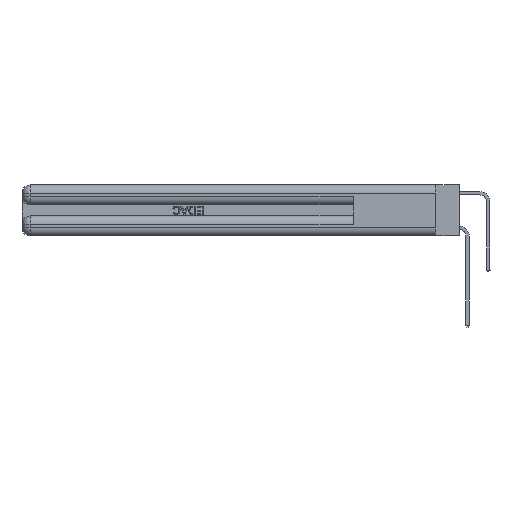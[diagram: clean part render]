
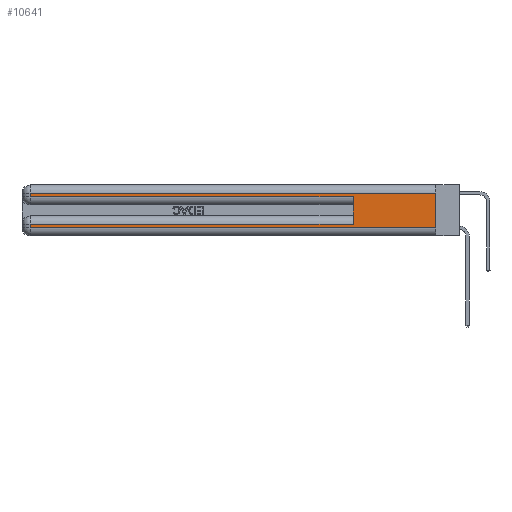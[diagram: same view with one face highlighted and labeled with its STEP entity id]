
A CAD part, left-side view. The second image highlights one B-rep face of the part: STEP entity #10641.
In plain terms, the highlighted planar face has unit normal (-1, 0, 0).
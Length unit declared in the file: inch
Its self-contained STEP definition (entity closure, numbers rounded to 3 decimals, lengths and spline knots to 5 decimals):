
#308 = PLANE ( 'NONE',  #33304 ) ;
#389 = VECTOR ( 'NONE', #32536, 39.37008 ) ;
#602 = DIRECTION ( 'NONE',  ( 0., 0., -1. ) ) ;
#953 = CARTESIAN_POINT ( 'NONE',  ( 0., 0.6, 0.145 ) ) ;
#1330 = CARTESIAN_POINT ( 'NONE',  ( 0., 0.6, 0.085 ) ) ;
#2052 = CARTESIAN_POINT ( 'NONE',  ( 0., 0.6, 0.285 ) ) ;
#2738 = ORIENTED_EDGE ( 'NONE', *, *, #14764, .T. ) ;
#3530 = DIRECTION ( 'NONE',  ( 0., 0., -1. ) ) ;
#4012 = LINE ( 'NONE', #33221, #389 ) ;
#4096 = CARTESIAN_POINT ( 'NONE',  ( 0., 0., 0.31 ) ) ;
#4951 = CARTESIAN_POINT ( 'NONE',  ( 0., 0., 0.31 ) ) ;
#5007 = EDGE_CURVE ( 'NONE', #8560, #24838, #16188, .T. ) ;
#5132 = DIRECTION ( 'NONE',  ( 0., 0., -1. ) ) ;
#6076 = CARTESIAN_POINT ( 'NONE',  ( 0., 0., 0.085 ) ) ;
#6157 = ORIENTED_EDGE ( 'NONE', *, *, #23378, .T. ) ;
#6647 = CARTESIAN_POINT ( 'NONE',  ( 0., 0., 0.06 ) ) ;
#7600 = VECTOR ( 'NONE', #22422, 39.37008 ) ;
#8117 = DIRECTION ( 'NONE',  ( 0., 1., 0. ) ) ;
#8440 = ORIENTED_EDGE ( 'NONE', *, *, #5007, .T. ) ;
#8560 = VERTEX_POINT ( 'NONE', #4951 ) ;
#9356 = LINE ( 'NONE', #32556, #15808 ) ;
#10148 = VECTOR ( 'NONE', #8117, 39.37008 ) ;
#10641 = ADVANCED_FACE ( 'NONE', ( #25925 ), #308, .F. ) ;
#10851 = ORIENTED_EDGE ( 'NONE', *, *, #27778, .T. ) ;
#11109 = DIRECTION ( 'NONE',  ( 0., -1., 0. ) ) ;
#11362 = EDGE_CURVE ( 'NONE', #14599, #24859, #4012, .T. ) ;
#11548 = LINE ( 'NONE', #6076, #19708 ) ;
#13136 = VERTEX_POINT ( 'NONE', #30619 ) ;
#14599 = VERTEX_POINT ( 'NONE', #21349 ) ;
#14764 = EDGE_CURVE ( 'NONE', #26136, #14599, #11548, .T. ) ;
#15808 = VECTOR ( 'NONE', #3530, 39.37008 ) ;
#16075 = LINE ( 'NONE', #24159, #30974 ) ;
#16188 = LINE ( 'NONE', #4096, #10148 ) ;
#16598 = CARTESIAN_POINT ( 'NONE',  ( 0., 0., 0.285 ) ) ;
#16610 = LINE ( 'NONE', #6647, #29931 ) ;
#18191 = DIRECTION ( 'NONE',  ( 1., 0., 0. ) ) ;
#19239 = VERTEX_POINT ( 'NONE', #2052 ) ;
#19510 = ORIENTED_EDGE ( 'NONE', *, *, #11362, .T. ) ;
#19708 = VECTOR ( 'NONE', #29935, 39.37008 ) ;
#19840 = CARTESIAN_POINT ( 'NONE',  ( 0., 2.94, 0.285 ) ) ;
#19963 = EDGE_CURVE ( 'NONE', #8560, #13136, #16075, .T. ) ;
#21205 = ORIENTED_EDGE ( 'NONE', *, *, #30192, .F. ) ;
#21305 = EDGE_LOOP ( 'NONE', ( #22334, #8440, #26235, #10851, #21205, #2738, #19510, #6157 ) ) ;
#21320 = VERTEX_POINT ( 'NONE', #19840 ) ;
#21349 = CARTESIAN_POINT ( 'NONE',  ( 0., 2.94, 0.085 ) ) ;
#21744 = DIRECTION ( 'NONE',  ( 0., 0., 1. ) ) ;
#22334 = ORIENTED_EDGE ( 'NONE', *, *, #19963, .F. ) ;
#22422 = DIRECTION ( 'NONE',  ( 0., -1., 0. ) ) ;
#23125 = CARTESIAN_POINT ( 'NONE',  ( 0., 2.94, 0.06 ) ) ;
#23352 = CARTESIAN_POINT ( 'NONE',  ( 0., 0., 0.37 ) ) ;
#23378 = EDGE_CURVE ( 'NONE', #24859, #13136, #16610, .T. ) ;
#23993 = LINE ( 'NONE', #953, #26350 ) ;
#24159 = CARTESIAN_POINT ( 'NONE',  ( 0., 0., 0.37 ) ) ;
#24838 = VERTEX_POINT ( 'NONE', #33432 ) ;
#24859 = VERTEX_POINT ( 'NONE', #23125 ) ;
#25925 = FACE_OUTER_BOUND ( 'NONE', #21305, .T. ) ;
#26136 = VERTEX_POINT ( 'NONE', #1330 ) ;
#26235 = ORIENTED_EDGE ( 'NONE', *, *, #27702, .T. ) ;
#26350 = VECTOR ( 'NONE', #21744, 39.37008 ) ;
#27702 = EDGE_CURVE ( 'NONE', #24838, #21320, #9356, .T. ) ;
#27778 = EDGE_CURVE ( 'NONE', #21320, #19239, #30158, .T. ) ;
#29931 = VECTOR ( 'NONE', #11109, 39.37008 ) ;
#29935 = DIRECTION ( 'NONE',  ( 0., 1., 0. ) ) ;
#30158 = LINE ( 'NONE', #16598, #7600 ) ;
#30192 = EDGE_CURVE ( 'NONE', #26136, #19239, #23993, .T. ) ;
#30619 = CARTESIAN_POINT ( 'NONE',  ( 0., 0., 0.06 ) ) ;
#30974 = VECTOR ( 'NONE', #602, 39.37008 ) ;
#32536 = DIRECTION ( 'NONE',  ( 0., 0., -1. ) ) ;
#32556 = CARTESIAN_POINT ( 'NONE',  ( 0., 2.94, 0.37 ) ) ;
#33221 = CARTESIAN_POINT ( 'NONE',  ( 0., 2.94, 0.37 ) ) ;
#33304 = AXIS2_PLACEMENT_3D ( 'NONE', #23352, #18191, #5132 ) ;
#33432 = CARTESIAN_POINT ( 'NONE',  ( 0., 2.94, 0.31 ) ) ;
